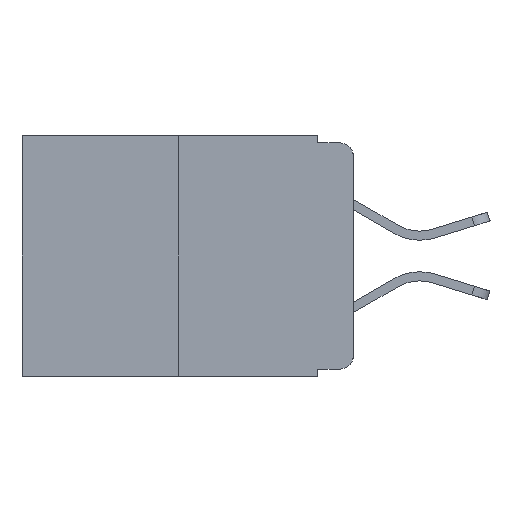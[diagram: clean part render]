
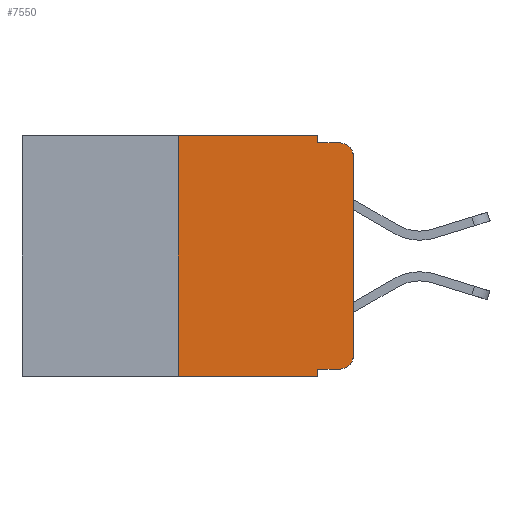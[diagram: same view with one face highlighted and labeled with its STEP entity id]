
A CAD part, left-side view. The second image highlights one B-rep face of the part: STEP entity #7550.
In plain terms, the highlighted planar face has unit normal (-1, 0, 0).
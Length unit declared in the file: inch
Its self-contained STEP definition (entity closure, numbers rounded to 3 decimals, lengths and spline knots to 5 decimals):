
#86 = LINE ( 'NONE', #8843, #10664 ) ;
#291 = VERTEX_POINT ( 'NONE', #17431 ) ;
#944 = LINE ( 'NONE', #17473, #7951 ) ;
#1034 = CIRCLE ( 'NONE', #23789, 0.02 ) ;
#1390 = ORIENTED_EDGE ( 'NONE', *, *, #25827, .T. ) ;
#2095 = DIRECTION ( 'NONE',  ( 0., 0., -1. ) ) ;
#2266 = DIRECTION ( 'NONE',  ( -1., 0., 0. ) ) ;
#2817 = DIRECTION ( 'NONE',  ( 1., 0., 0. ) ) ;
#3358 = ORIENTED_EDGE ( 'NONE', *, *, #6197, .F. ) ;
#3377 = VERTEX_POINT ( 'NONE', #13430 ) ;
#4132 = AXIS2_PLACEMENT_3D ( 'NONE', #25626, #7363, #17377 ) ;
#4310 = DIRECTION ( 'NONE',  ( 0., 0., -1. ) ) ;
#4321 = EDGE_CURVE ( 'NONE', #22790, #25672, #12176, .T. ) ;
#4690 = CARTESIAN_POINT ( 'NONE',  ( 0., 0.473, -0.343 ) ) ;
#5065 = ORIENTED_EDGE ( 'NONE', *, *, #22250, .T. ) ;
#5266 = VECTOR ( 'NONE', #9152, 39.37008 ) ;
#5516 = EDGE_CURVE ( 'NONE', #9880, #3377, #23220, .T. ) ;
#5574 = VECTOR ( 'NONE', #25410, 39.37008 ) ;
#6197 = EDGE_CURVE ( 'NONE', #25672, #9880, #22552, .T. ) ;
#6269 = CARTESIAN_POINT ( 'NONE',  ( 0., 0.02, -0.333 ) ) ;
#6415 = VERTEX_POINT ( 'NONE', #19102 ) ;
#6927 = CARTESIAN_POINT ( 'NONE',  ( 0., 0., -0.03 ) ) ;
#6965 = CARTESIAN_POINT ( 'NONE',  ( 0., 0., 0. ) ) ;
#7127 = VERTEX_POINT ( 'NONE', #6927 ) ;
#7363 = DIRECTION ( 'NONE',  ( -1., 0., 0. ) ) ;
#7550 = ADVANCED_FACE ( 'NONE', ( #10395 ), #13158, .F. ) ;
#7951 = VECTOR ( 'NONE', #9255, 39.37008 ) ;
#8252 = ORIENTED_EDGE ( 'NONE', *, *, #22145, .F. ) ;
#8380 = ORIENTED_EDGE ( 'NONE', *, *, #10100, .T. ) ;
#8725 = CARTESIAN_POINT ( 'NONE',  ( 0., 0., -0.313 ) ) ;
#8843 = CARTESIAN_POINT ( 'NONE',  ( 0., 0.051, -0.333 ) ) ;
#9152 = DIRECTION ( 'NONE',  ( 0., 0., 1. ) ) ;
#9255 = DIRECTION ( 'NONE',  ( 0., 0., -1. ) ) ;
#9707 = EDGE_CURVE ( 'NONE', #291, #21337, #86, .T. ) ;
#9865 = CARTESIAN_POINT ( 'NONE',  ( 0., 0.051, 0. ) ) ;
#9880 = VERTEX_POINT ( 'NONE', #17518 ) ;
#10100 = EDGE_CURVE ( 'NONE', #7127, #3377, #1034, .T. ) ;
#10395 = FACE_OUTER_BOUND ( 'NONE', #12653, .T. ) ;
#10528 = ORIENTED_EDGE ( 'NONE', *, *, #16991, .T. ) ;
#10664 = VECTOR ( 'NONE', #21350, 39.37008 ) ;
#11019 = LINE ( 'NONE', #6965, #5574 ) ;
#11800 = VERTEX_POINT ( 'NONE', #21509 ) ;
#12176 = LINE ( 'NONE', #12411, #12810 ) ;
#12334 = LINE ( 'NONE', #19604, #5266 ) ;
#12411 = CARTESIAN_POINT ( 'NONE',  ( 0., 0.473, 0. ) ) ;
#12439 = VECTOR ( 'NONE', #18976, 39.37008 ) ;
#12653 = EDGE_LOOP ( 'NONE', ( #10528, #8380, #22923, #3358, #24383, #8252, #1390, #26012, #21014, #5065 ) ) ;
#12810 = VECTOR ( 'NONE', #14273, 39.37008 ) ;
#13158 = PLANE ( 'NONE',  #13218 ) ;
#13218 = AXIS2_PLACEMENT_3D ( 'NONE', #16842, #2817, #23274 ) ;
#13430 = CARTESIAN_POINT ( 'NONE',  ( 0., 0.02, -0.01 ) ) ;
#13443 = CARTESIAN_POINT ( 'NONE',  ( 0., 0.051, -0.01 ) ) ;
#13693 = VECTOR ( 'NONE', #23294, 39.37008 ) ;
#14273 = DIRECTION ( 'NONE',  ( 0., -1., 0. ) ) ;
#14939 = CARTESIAN_POINT ( 'NONE',  ( 0., 0.25, 0. ) ) ;
#15922 = LINE ( 'NONE', #4690, #12439 ) ;
#16186 = CARTESIAN_POINT ( 'NONE',  ( 0., 0.051, 0. ) ) ;
#16842 = CARTESIAN_POINT ( 'NONE',  ( 0., 0.473, 0. ) ) ;
#16991 = EDGE_CURVE ( 'NONE', #24617, #7127, #11019, .T. ) ;
#17377 = DIRECTION ( 'NONE',  ( 0., 0., -1. ) ) ;
#17431 = CARTESIAN_POINT ( 'NONE',  ( 0., 0.051, -0.333 ) ) ;
#17473 = CARTESIAN_POINT ( 'NONE',  ( 0., 0.051, 0. ) ) ;
#17518 = CARTESIAN_POINT ( 'NONE',  ( 0., 0.051, -0.01 ) ) ;
#18976 = DIRECTION ( 'NONE',  ( 0., -1., 0. ) ) ;
#19001 = EDGE_CURVE ( 'NONE', #291, #6415, #944, .T. ) ;
#19102 = CARTESIAN_POINT ( 'NONE',  ( 0., 0.051, -0.343 ) ) ;
#19604 = CARTESIAN_POINT ( 'NONE',  ( 0., 0.25, 0. ) ) ;
#21014 = ORIENTED_EDGE ( 'NONE', *, *, #9707, .T. ) ;
#21337 = VERTEX_POINT ( 'NONE', #6269 ) ;
#21350 = DIRECTION ( 'NONE',  ( 0., -1., 0. ) ) ;
#21509 = CARTESIAN_POINT ( 'NONE',  ( 0., 0.25, -0.343 ) ) ;
#21629 = VECTOR ( 'NONE', #2095, 39.37008 ) ;
#22145 = EDGE_CURVE ( 'NONE', #11800, #22790, #12334, .T. ) ;
#22250 = EDGE_CURVE ( 'NONE', #21337, #24617, #25977, .T. ) ;
#22552 = LINE ( 'NONE', #16186, #21629 ) ;
#22790 = VERTEX_POINT ( 'NONE', #14939 ) ;
#22923 = ORIENTED_EDGE ( 'NONE', *, *, #5516, .F. ) ;
#23220 = LINE ( 'NONE', #13443, #13693 ) ;
#23274 = DIRECTION ( 'NONE',  ( 0., 0., -1. ) ) ;
#23294 = DIRECTION ( 'NONE',  ( 0., -1., 0. ) ) ;
#23789 = AXIS2_PLACEMENT_3D ( 'NONE', #24428, #2266, #4310 ) ;
#24383 = ORIENTED_EDGE ( 'NONE', *, *, #4321, .F. ) ;
#24428 = CARTESIAN_POINT ( 'NONE',  ( 0., 0.02, -0.03 ) ) ;
#24617 = VERTEX_POINT ( 'NONE', #8725 ) ;
#25410 = DIRECTION ( 'NONE',  ( 0., 0., 1. ) ) ;
#25626 = CARTESIAN_POINT ( 'NONE',  ( 0., 0.02, -0.313 ) ) ;
#25672 = VERTEX_POINT ( 'NONE', #9865 ) ;
#25827 = EDGE_CURVE ( 'NONE', #11800, #6415, #15922, .T. ) ;
#25977 = CIRCLE ( 'NONE', #4132, 0.02 ) ;
#26012 = ORIENTED_EDGE ( 'NONE', *, *, #19001, .F. ) ;
